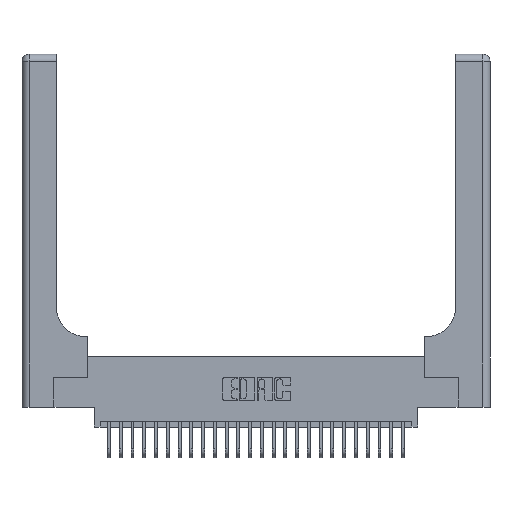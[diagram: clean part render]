
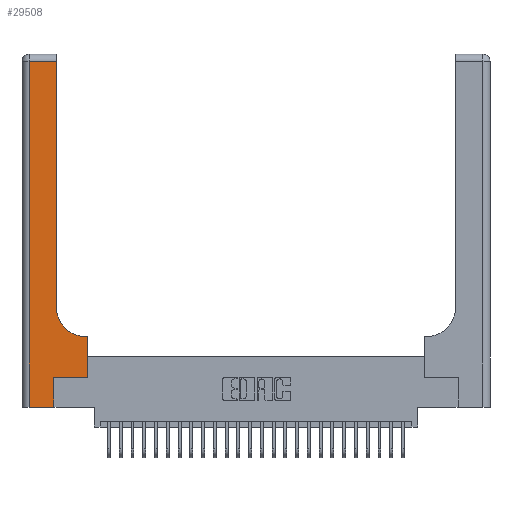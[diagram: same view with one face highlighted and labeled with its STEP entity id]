
A CAD part, top view. The second image highlights one B-rep face of the part: STEP entity #29508.
In plain terms, the highlighted planar face has unit normal (0, 0, 1).
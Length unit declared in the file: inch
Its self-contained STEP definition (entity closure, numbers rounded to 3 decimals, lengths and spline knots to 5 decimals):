
#420 = DIRECTION ( 'NONE',  ( 0., 1., 0. ) ) ;
#825 = VECTOR ( 'NONE', #24550, 39.37008 ) ;
#903 = DIRECTION ( 'NONE',  ( 0., 1., 0. ) ) ;
#986 = VECTOR ( 'NONE', #10392, 39.37008 ) ;
#1014 = CARTESIAN_POINT ( 'NONE',  ( 0.5585, 0.25, 0.37 ) ) ;
#1248 = CARTESIAN_POINT ( 'NONE',  ( 0.2915, 0.85, 0.37 ) ) ;
#1307 = CARTESIAN_POINT ( 'NONE',  ( 0., 3., 0.37 ) ) ;
#1370 = VECTOR ( 'NONE', #4524, 39.37008 ) ;
#1840 = EDGE_CURVE ( 'NONE', #20834, #14370, #20473, .T. ) ;
#2382 = LINE ( 'NONE', #19358, #25973 ) ;
#2664 = EDGE_CURVE ( 'NONE', #13703, #4546, #8328, .T. ) ;
#3345 = LINE ( 'NONE', #1014, #13419 ) ;
#3488 = VERTEX_POINT ( 'NONE', #14952 ) ;
#3701 = DIRECTION ( 'NONE',  ( -1., 0., 0. ) ) ;
#4209 = DIRECTION ( 'NONE',  ( -1., 0., 0. ) ) ;
#4524 = DIRECTION ( 'NONE',  ( 1., 0., 0. ) ) ;
#4546 = VERTEX_POINT ( 'NONE', #16423 ) ;
#4785 = VECTOR ( 'NONE', #4209, 39.37008 ) ;
#5335 = AXIS2_PLACEMENT_3D ( 'NONE', #1307, #17474, #3701 ) ;
#5416 = EDGE_CURVE ( 'NONE', #28510, #3488, #3345, .T. ) ;
#5700 = ORIENTED_EDGE ( 'NONE', *, *, #22689, .T. ) ;
#5807 = ORIENTED_EDGE ( 'NONE', *, *, #2664, .T. ) ;
#6302 = CARTESIAN_POINT ( 'NONE',  ( 0.2915, 0.6, 0.37 ) ) ;
#6320 = LINE ( 'NONE', #6302, #825 ) ;
#8328 = LINE ( 'NONE', #27809, #19757 ) ;
#8968 = CARTESIAN_POINT ( 'NONE',  ( 0.5415, 0.6, 0.37 ) ) ;
#9076 = CARTESIAN_POINT ( 'NONE',  ( 0.269, 0., 0.37 ) ) ;
#10392 = DIRECTION ( 'NONE',  ( 0., -1., 0. ) ) ;
#10709 = CARTESIAN_POINT ( 'NONE',  ( 0.06, 0., 0.37 ) ) ;
#10885 = LINE ( 'NONE', #29091, #4785 ) ;
#10978 = VERTEX_POINT ( 'NONE', #12902 ) ;
#11260 = ORIENTED_EDGE ( 'NONE', *, *, #17653, .T. ) ;
#11887 = CARTESIAN_POINT ( 'NONE',  ( 0.5415, 0.85, 0.37 ) ) ;
#12183 = ORIENTED_EDGE ( 'NONE', *, *, #23415, .T. ) ;
#12321 = EDGE_CURVE ( 'NONE', #10978, #28510, #20205, .T. ) ;
#12512 = ORIENTED_EDGE ( 'NONE', *, *, #26419, .T. ) ;
#12853 = PLANE ( 'NONE',  #5335 ) ;
#12902 = CARTESIAN_POINT ( 'NONE',  ( 0.269, 0.25, 0.37 ) ) ;
#13419 = VECTOR ( 'NONE', #28347, 39.37008 ) ;
#13703 = VERTEX_POINT ( 'NONE', #1248 ) ;
#14166 = DIRECTION ( 'NONE',  ( 1., 0., 0. ) ) ;
#14333 = VERTEX_POINT ( 'NONE', #8968 ) ;
#14370 = VERTEX_POINT ( 'NONE', #9076 ) ;
#14442 = ORIENTED_EDGE ( 'NONE', *, *, #12321, .T. ) ;
#14952 = CARTESIAN_POINT ( 'NONE',  ( 0.5585, 0.6, 0.37 ) ) ;
#14964 = CARTESIAN_POINT ( 'NONE',  ( 0.06, 3., 0.37 ) ) ;
#15302 = ORIENTED_EDGE ( 'NONE', *, *, #27871, .T. ) ;
#16423 = CARTESIAN_POINT ( 'NONE',  ( 0.2915, 2.94, 0.37 ) ) ;
#17121 = VERTEX_POINT ( 'NONE', #26458 ) ;
#17474 = DIRECTION ( 'NONE',  ( 0., 0., -1. ) ) ;
#17653 = EDGE_CURVE ( 'NONE', #14370, #10978, #2382, .T. ) ;
#17941 = CARTESIAN_POINT ( 'NONE',  ( 0.269, 0.25, 0.37 ) ) ;
#18338 = AXIS2_PLACEMENT_3D ( 'NONE', #11887, #27678, #14166 ) ;
#19358 = CARTESIAN_POINT ( 'NONE',  ( 0.269, 0., 0.37 ) ) ;
#19406 = EDGE_LOOP ( 'NONE', ( #5807, #12183, #5700, #21748, #11260, #14442, #27429, #15302, #12512 ) ) ;
#19482 = VECTOR ( 'NONE', #20224, 39.37008 ) ;
#19757 = VECTOR ( 'NONE', #420, 39.37008 ) ;
#20205 = LINE ( 'NONE', #17941, #19482 ) ;
#20224 = DIRECTION ( 'NONE',  ( 1., 0., 0. ) ) ;
#20473 = LINE ( 'NONE', #20555, #1370 ) ;
#20555 = CARTESIAN_POINT ( 'NONE',  ( 0., 0., 0.37 ) ) ;
#20834 = VERTEX_POINT ( 'NONE', #10709 ) ;
#21748 = ORIENTED_EDGE ( 'NONE', *, *, #1840, .T. ) ;
#22282 = CARTESIAN_POINT ( 'NONE',  ( 0.5585, 0.25, 0.37 ) ) ;
#22689 = EDGE_CURVE ( 'NONE', #17121, #20834, #26066, .T. ) ;
#23403 = FACE_OUTER_BOUND ( 'NONE', #19406, .T. ) ;
#23415 = EDGE_CURVE ( 'NONE', #4546, #17121, #10885, .T. ) ;
#24550 = DIRECTION ( 'NONE',  ( -1., 0., 0. ) ) ;
#25973 = VECTOR ( 'NONE', #903, 39.37008 ) ;
#26066 = LINE ( 'NONE', #14964, #986 ) ;
#26419 = EDGE_CURVE ( 'NONE', #14333, #13703, #26973, .T. ) ;
#26458 = CARTESIAN_POINT ( 'NONE',  ( 0.06, 2.94, 0.37 ) ) ;
#26973 = CIRCLE ( 'NONE', #18338, 0.25 ) ;
#27429 = ORIENTED_EDGE ( 'NONE', *, *, #5416, .T. ) ;
#27678 = DIRECTION ( 'NONE',  ( 0., 0., -1. ) ) ;
#27809 = CARTESIAN_POINT ( 'NONE',  ( 0.2915, 3., 0.37 ) ) ;
#27871 = EDGE_CURVE ( 'NONE', #3488, #14333, #6320, .T. ) ;
#28347 = DIRECTION ( 'NONE',  ( 0., 1., 0. ) ) ;
#28510 = VERTEX_POINT ( 'NONE', #22282 ) ;
#29091 = CARTESIAN_POINT ( 'NONE',  ( 0., 2.94, 0.37 ) ) ;
#29508 = ADVANCED_FACE ( 'NONE', ( #23403 ), #12853, .F. ) ;
